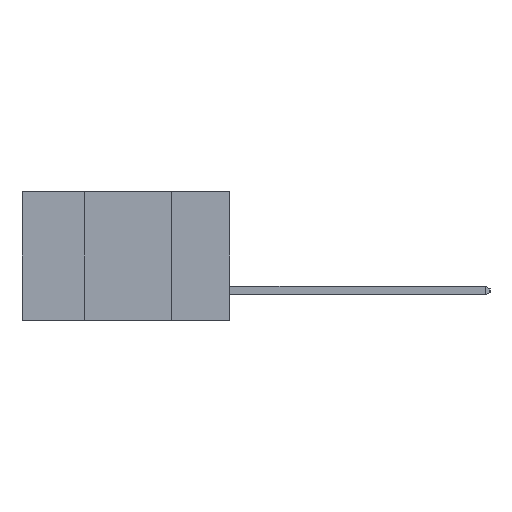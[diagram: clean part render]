
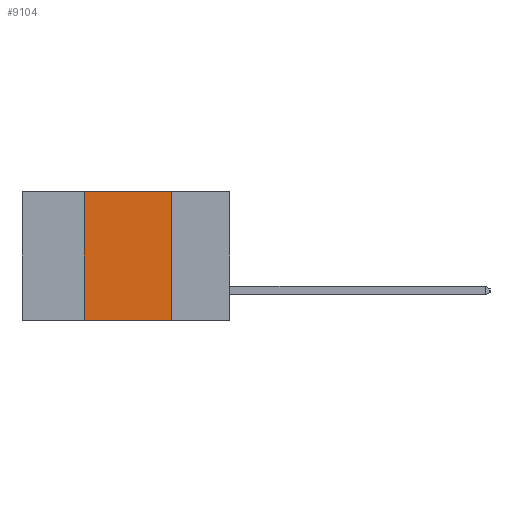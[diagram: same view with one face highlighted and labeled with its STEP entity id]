
A CAD part, left-side view. The second image highlights one B-rep face of the part: STEP entity #9104.
In plain terms, the highlighted planar face has unit normal (-1, 0, 0).
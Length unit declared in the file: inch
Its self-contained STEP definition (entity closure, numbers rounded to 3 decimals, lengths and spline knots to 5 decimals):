
#121 = CARTESIAN_POINT ( 'NONE',  ( 0., 0.6, -0.37 ) ) ;
#204 = ORIENTED_EDGE ( 'NONE', *, *, #12042, .F. ) ;
#342 = DIRECTION ( 'NONE',  ( 0., 0., -1. ) ) ;
#721 = LINE ( 'NONE', #11496, #7787 ) ;
#797 = CARTESIAN_POINT ( 'NONE',  ( 0., 0.42, 0. ) ) ;
#1099 = ORIENTED_EDGE ( 'NONE', *, *, #12917, .T. ) ;
#1197 = EDGE_LOOP ( 'NONE', ( #5246, #9010, #204, #1099 ) ) ;
#1329 = DIRECTION ( 'NONE',  ( 0., 0., -1. ) ) ;
#1460 = VECTOR ( 'NONE', #1329, 39.37008 ) ;
#1463 = VERTEX_POINT ( 'NONE', #14875 ) ;
#4571 = PLANE ( 'NONE',  #11248 ) ;
#5246 = ORIENTED_EDGE ( 'NONE', *, *, #9542, .F. ) ;
#5684 = FACE_OUTER_BOUND ( 'NONE', #1197, .T. ) ;
#5830 = DIRECTION ( 'NONE',  ( 0., -1., 0. ) ) ;
#6011 = DIRECTION ( 'NONE',  ( 0., -1., 0. ) ) ;
#6467 = CARTESIAN_POINT ( 'NONE',  ( 0., 0.42, -0.37 ) ) ;
#7377 = CARTESIAN_POINT ( 'NONE',  ( 0., 0.6, 0. ) ) ;
#7679 = DIRECTION ( 'NONE',  ( 0., 0., 1. ) ) ;
#7787 = VECTOR ( 'NONE', #6011, 39.37008 ) ;
#8354 = CARTESIAN_POINT ( 'NONE',  ( 0., 0.17, -0.37 ) ) ;
#8493 = LINE ( 'NONE', #8354, #1460 ) ;
#8779 = DIRECTION ( 'NONE',  ( 1., 0., 0. ) ) ;
#9010 = ORIENTED_EDGE ( 'NONE', *, *, #11147, .F. ) ;
#9104 = ADVANCED_FACE ( 'NONE', ( #5684 ), #4571, .F. ) ;
#9475 = LINE ( 'NONE', #13067, #15717 ) ;
#9542 = EDGE_CURVE ( 'NONE', #12905, #1463, #8493, .T. ) ;
#10718 = VERTEX_POINT ( 'NONE', #6467 ) ;
#10940 = VECTOR ( 'NONE', #5830, 39.37008 ) ;
#11147 = EDGE_CURVE ( 'NONE', #13270, #12905, #721, .T. ) ;
#11248 = AXIS2_PLACEMENT_3D ( 'NONE', #7377, #8779, #342 ) ;
#11496 = CARTESIAN_POINT ( 'NONE',  ( 0., 0.6, 0. ) ) ;
#12042 = EDGE_CURVE ( 'NONE', #10718, #13270, #9475, .T. ) ;
#12905 = VERTEX_POINT ( 'NONE', #15239 ) ;
#12917 = EDGE_CURVE ( 'NONE', #10718, #1463, #14882, .T. ) ;
#13067 = CARTESIAN_POINT ( 'NONE',  ( 0., 0.42, -0.37 ) ) ;
#13270 = VERTEX_POINT ( 'NONE', #797 ) ;
#14875 = CARTESIAN_POINT ( 'NONE',  ( 0., 0.17, -0.37 ) ) ;
#14882 = LINE ( 'NONE', #121, #10940 ) ;
#15239 = CARTESIAN_POINT ( 'NONE',  ( 0., 0.17, 0. ) ) ;
#15717 = VECTOR ( 'NONE', #7679, 39.37008 ) ;
